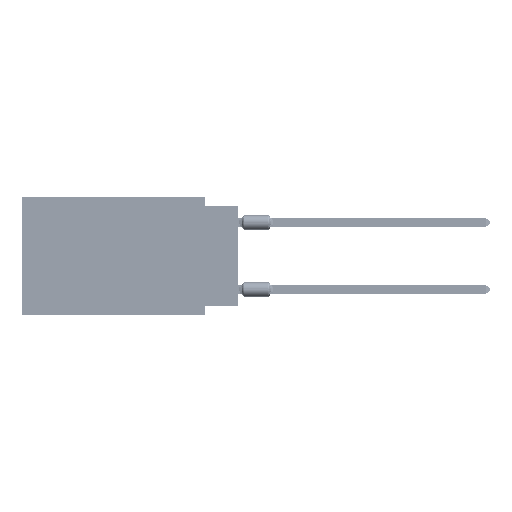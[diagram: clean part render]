
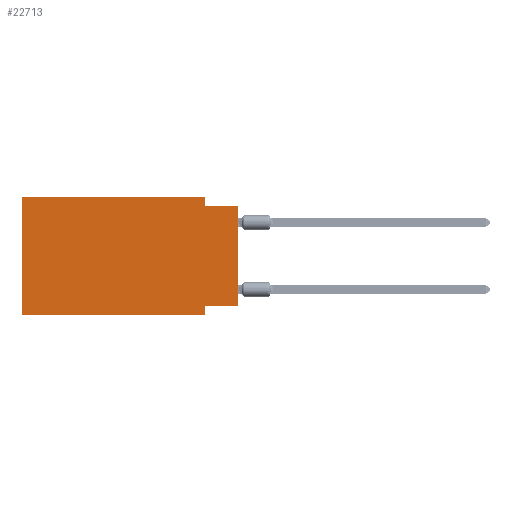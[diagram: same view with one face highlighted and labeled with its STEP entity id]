
A CAD part, left-side view. The second image highlights one B-rep face of the part: STEP entity #22713.
In plain terms, the highlighted planar face has unit normal (-1, 0, 0).
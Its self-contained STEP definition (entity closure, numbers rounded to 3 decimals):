
#192 = DIRECTION ( 'NONE',  ( 0., 0., -1. ) ) ;
#1171 = DIRECTION ( 'NONE',  ( 0., -1., 0. ) ) ;
#3288 = VECTOR ( 'NONE', #65954, 1000. ) ;
#3432 = CARTESIAN_POINT ( 'NONE',  ( 0., 2.54, 0. ) ) ;
#3964 = DIRECTION ( 'NONE',  ( 0., 0., -1. ) ) ;
#5365 = CARTESIAN_POINT ( 'NONE',  ( 0., 2.54, -8.255 ) ) ;
#8439 = CARTESIAN_POINT ( 'NONE',  ( 0., 2.54, -8.89 ) ) ;
#9247 = EDGE_CURVE ( 'NONE', #49192, #36090, #55109, .T. ) ;
#11827 = CARTESIAN_POINT ( 'NONE',  ( 0., 0., -8.255 ) ) ;
#13462 = VERTEX_POINT ( 'NONE', #48324 ) ;
#13590 = CARTESIAN_POINT ( 'NONE',  ( 0., 16.383, 0. ) ) ;
#16484 = EDGE_CURVE ( 'NONE', #69592, #28417, #35632, .T. ) ;
#17258 = CARTESIAN_POINT ( 'NONE',  ( 0., 0., -0.635 ) ) ;
#17404 = ORIENTED_EDGE ( 'NONE', *, *, #53411, .T. ) ;
#20976 = ORIENTED_EDGE ( 'NONE', *, *, #62379, .F. ) ;
#22130 = DIRECTION ( 'NONE',  ( 0., -1., 0. ) ) ;
#22504 = CARTESIAN_POINT ( 'NONE',  ( 0., 0., -0.635 ) ) ;
#22620 = CARTESIAN_POINT ( 'NONE',  ( 0., 16.383, -8.89 ) ) ;
#22713 = ADVANCED_FACE ( 'NONE', ( #60733 ), #48776, .F. ) ;
#22868 = CARTESIAN_POINT ( 'NONE',  ( 0., 0., 0. ) ) ;
#23914 = VECTOR ( 'NONE', #62435, 1000. ) ;
#28245 = ORIENTED_EDGE ( 'NONE', *, *, #9247, .F. ) ;
#28417 = VERTEX_POINT ( 'NONE', #36265 ) ;
#28863 = ORIENTED_EDGE ( 'NONE', *, *, #53417, .F. ) ;
#30063 = EDGE_LOOP ( 'NONE', ( #17404, #28863, #41441, #65531, #52376, #33914, #20976, #28245 ) ) ;
#30207 = DIRECTION ( 'NONE',  ( 0., 0., -1. ) ) ;
#30414 = VECTOR ( 'NONE', #41958, 1000. ) ;
#31312 = LINE ( 'NONE', #59686, #57261 ) ;
#31387 = CARTESIAN_POINT ( 'NONE',  ( 0., 16.383, -8.89 ) ) ;
#33880 = VECTOR ( 'NONE', #1171, 1000. ) ;
#33914 = ORIENTED_EDGE ( 'NONE', *, *, #56837, .T. ) ;
#34349 = EDGE_CURVE ( 'NONE', #28417, #43288, #63549, .T. ) ;
#35632 = LINE ( 'NONE', #13590, #30414 ) ;
#36090 = VERTEX_POINT ( 'NONE', #5365 ) ;
#36265 = CARTESIAN_POINT ( 'NONE',  ( 0., 16.383, 0. ) ) ;
#38308 = DIRECTION ( 'NONE',  ( 1., 0., 0. ) ) ;
#41441 = ORIENTED_EDGE ( 'NONE', *, *, #68878, .F. ) ;
#41958 = DIRECTION ( 'NONE',  ( 0., 0., 1. ) ) ;
#43288 = VERTEX_POINT ( 'NONE', #3432 ) ;
#43534 = CARTESIAN_POINT ( 'NONE',  ( 0., 16.383, 0. ) ) ;
#45987 = LINE ( 'NONE', #22868, #23914 ) ;
#46730 = CARTESIAN_POINT ( 'NONE',  ( 0., 16.383, 0. ) ) ;
#47274 = AXIS2_PLACEMENT_3D ( 'NONE', #43534, #38308, #3964 ) ;
#48324 = CARTESIAN_POINT ( 'NONE',  ( 0., 2.54, -0.635 ) ) ;
#48776 = PLANE ( 'NONE',  #47274 ) ;
#49192 = VERTEX_POINT ( 'NONE', #11827 ) ;
#49860 = CARTESIAN_POINT ( 'NONE',  ( 0., 2.54, -8.89 ) ) ;
#51660 = VECTOR ( 'NONE', #60137, 1000. ) ;
#52216 = VECTOR ( 'NONE', #192, 1000. ) ;
#52376 = ORIENTED_EDGE ( 'NONE', *, *, #16484, .F. ) ;
#53411 = EDGE_CURVE ( 'NONE', #49192, #69923, #45987, .T. ) ;
#53417 = EDGE_CURVE ( 'NONE', #13462, #69923, #63175, .T. ) ;
#55109 = LINE ( 'NONE', #70809, #3288 ) ;
#56837 = EDGE_CURVE ( 'NONE', #69592, #62239, #59765, .T. ) ;
#57261 = VECTOR ( 'NONE', #30207, 1000. ) ;
#59686 = CARTESIAN_POINT ( 'NONE',  ( 0., 2.54, 0. ) ) ;
#59765 = LINE ( 'NONE', #31387, #51660 ) ;
#60137 = DIRECTION ( 'NONE',  ( 0., -1., 0. ) ) ;
#60733 = FACE_OUTER_BOUND ( 'NONE', #30063, .T. ) ;
#62239 = VERTEX_POINT ( 'NONE', #8439 ) ;
#62379 = EDGE_CURVE ( 'NONE', #36090, #62239, #67037, .T. ) ;
#62435 = DIRECTION ( 'NONE',  ( 0., 0., 1. ) ) ;
#63175 = LINE ( 'NONE', #22504, #65638 ) ;
#63549 = LINE ( 'NONE', #46730, #33880 ) ;
#65531 = ORIENTED_EDGE ( 'NONE', *, *, #34349, .F. ) ;
#65638 = VECTOR ( 'NONE', #22130, 1000. ) ;
#65954 = DIRECTION ( 'NONE',  ( 0., 1., 0. ) ) ;
#67037 = LINE ( 'NONE', #49860, #52216 ) ;
#68878 = EDGE_CURVE ( 'NONE', #43288, #13462, #31312, .T. ) ;
#69592 = VERTEX_POINT ( 'NONE', #22620 ) ;
#69923 = VERTEX_POINT ( 'NONE', #17258 ) ;
#70809 = CARTESIAN_POINT ( 'NONE',  ( 0., 0., -8.255 ) ) ;
